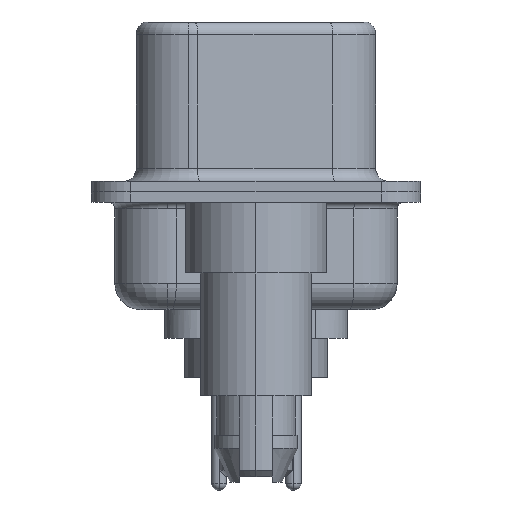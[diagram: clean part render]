
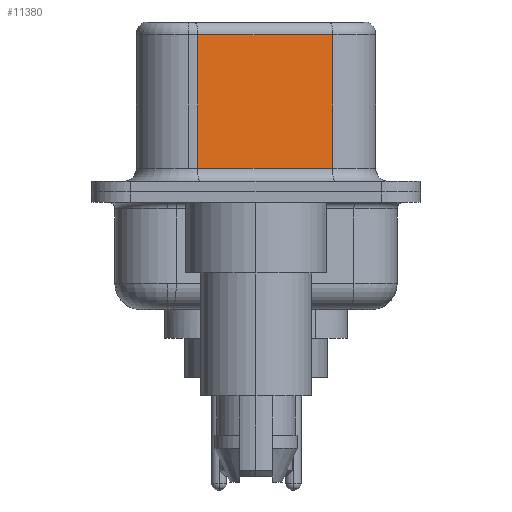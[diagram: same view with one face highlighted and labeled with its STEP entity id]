
A CAD part, left-side view. The second image highlights one B-rep face of the part: STEP entity #11380.
In plain terms, the highlighted planar face has unit normal (-0.985, -0.174, 0).
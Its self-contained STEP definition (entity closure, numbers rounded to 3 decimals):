
#653 = FACE_OUTER_BOUND ( 'NONE', #4853, .T. ) ;
#703 = ORIENTED_EDGE ( 'NONE', *, *, #11960, .F. ) ;
#987 = VERTEX_POINT ( 'NONE', #1462 ) ;
#1462 = CARTESIAN_POINT ( 'NONE',  ( 3.675, 2.233, 6.02 ) ) ;
#2268 = LINE ( 'NONE', #11349, #9133 ) ;
#2679 = CARTESIAN_POINT ( 'NONE',  ( 4.585, -2.927, 6.52 ) ) ;
#3135 = VERTEX_POINT ( 'NONE', #16133 ) ;
#3230 = CARTESIAN_POINT ( 'NONE',  ( 4.585, -2.927, 6.02 ) ) ;
#4048 = VECTOR ( 'NONE', #11538, 1000. ) ;
#4853 = EDGE_LOOP ( 'NONE', ( #703, #11715, #16386, #11493 ) ) ;
#5168 = CARTESIAN_POINT ( 'NONE',  ( 4.585, -2.927, 6.52 ) ) ;
#5251 = AXIS2_PLACEMENT_3D ( 'NONE', #5168, #15037, #6569 ) ;
#6569 = DIRECTION ( 'NONE',  ( -0.174, 0.985, 0. ) ) ;
#6669 = LINE ( 'NONE', #2679, #17863 ) ;
#7225 = VERTEX_POINT ( 'NONE', #16713 ) ;
#7661 = VERTEX_POINT ( 'NONE', #11603 ) ;
#7921 = CARTESIAN_POINT ( 'NONE',  ( 4.585, -2.927, 0.9 ) ) ;
#8864 = EDGE_CURVE ( 'NONE', #987, #7661, #2268, .T. ) ;
#9133 = VECTOR ( 'NONE', #9930, 1000. ) ;
#9331 = DIRECTION ( 'NONE',  ( 0.174, -0.985, 0. ) ) ;
#9930 = DIRECTION ( 'NONE',  ( 0., 0., -1. ) ) ;
#10386 = VECTOR ( 'NONE', #9331, 1000. ) ;
#10540 = EDGE_CURVE ( 'NONE', #7661, #3135, #14211, .T. ) ;
#11138 = EDGE_CURVE ( 'NONE', #7225, #987, #11894, .T. ) ;
#11349 = CARTESIAN_POINT ( 'NONE',  ( 3.675, 2.233, 6.52 ) ) ;
#11380 = ADVANCED_FACE ( 'NONE', ( #653 ), #13590, .F. ) ;
#11493 = ORIENTED_EDGE ( 'NONE', *, *, #10540, .T. ) ;
#11538 = DIRECTION ( 'NONE',  ( -0.174, 0.985, 0. ) ) ;
#11603 = CARTESIAN_POINT ( 'NONE',  ( 3.675, 2.233, 0.9 ) ) ;
#11715 = ORIENTED_EDGE ( 'NONE', *, *, #11138, .T. ) ;
#11894 = LINE ( 'NONE', #3230, #4048 ) ;
#11960 = EDGE_CURVE ( 'NONE', #7225, #3135, #6669, .T. ) ;
#13590 = PLANE ( 'NONE',  #5251 ) ;
#14211 = LINE ( 'NONE', #7921, #10386 ) ;
#15037 = DIRECTION ( 'NONE',  ( 0.985, 0.174, 0. ) ) ;
#15302 = DIRECTION ( 'NONE',  ( 0., 0., -1. ) ) ;
#16133 = CARTESIAN_POINT ( 'NONE',  ( 4.585, -2.927, 0.9 ) ) ;
#16386 = ORIENTED_EDGE ( 'NONE', *, *, #8864, .T. ) ;
#16713 = CARTESIAN_POINT ( 'NONE',  ( 4.585, -2.927, 6.02 ) ) ;
#17863 = VECTOR ( 'NONE', #15302, 1000. ) ;
